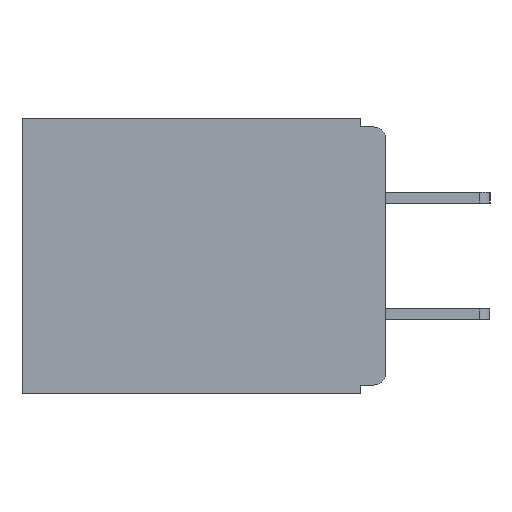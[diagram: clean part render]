
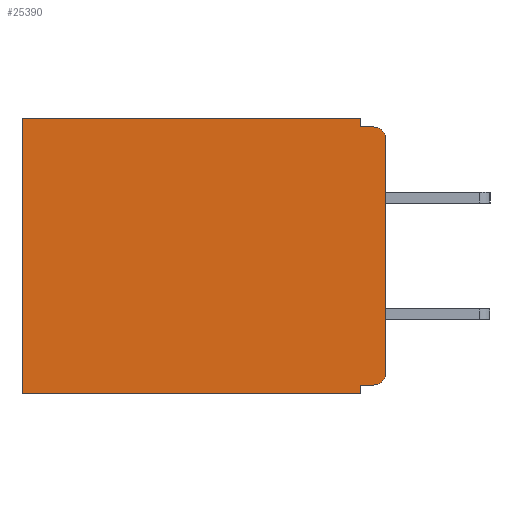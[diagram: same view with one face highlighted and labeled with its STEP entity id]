
A CAD part, left-side view. The second image highlights one B-rep face of the part: STEP entity #25390.
In plain terms, the highlighted planar face has unit normal (-1, 0, 0).
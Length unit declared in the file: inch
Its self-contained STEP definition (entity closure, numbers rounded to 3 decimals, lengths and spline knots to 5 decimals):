
#150 = DIRECTION ( 'NONE',  ( 0., 0., -1. ) ) ;
#1363 = VERTEX_POINT ( 'NONE', #24189 ) ;
#1389 = EDGE_CURVE ( 'NONE', #25102, #22044, #20073, .T. ) ;
#1518 = ORIENTED_EDGE ( 'NONE', *, *, #18378, .T. ) ;
#1550 = EDGE_CURVE ( 'NONE', #19092, #3243, #11316, .T. ) ;
#2679 = DIRECTION ( 'NONE',  ( 1., 0., 0. ) ) ;
#3073 = LINE ( 'NONE', #3217, #8347 ) ;
#3217 = CARTESIAN_POINT ( 'NONE',  ( 0.3, 0., -0.32 ) ) ;
#3243 = VERTEX_POINT ( 'NONE', #17066 ) ;
#3427 = VERTEX_POINT ( 'NONE', #26050 ) ;
#3461 = CIRCLE ( 'NONE', #15539, 0.015 ) ;
#4705 = CARTESIAN_POINT ( 'NONE',  ( 0.3, 0.015, -0.305 ) ) ;
#5525 = DIRECTION ( 'NONE',  ( 0., 1., 0. ) ) ;
#5981 = ORIENTED_EDGE ( 'NONE', *, *, #15393, .T. ) ;
#6112 = VECTOR ( 'NONE', #9221, 39.37008 ) ;
#6397 = DIRECTION ( 'NONE',  ( -1., 0., 0. ) ) ;
#6559 = ORIENTED_EDGE ( 'NONE', *, *, #17235, .T. ) ;
#6800 = CARTESIAN_POINT ( 'NONE',  ( 0.3, 0.031, -0.33 ) ) ;
#6948 = DIRECTION ( 'NONE',  ( 0., 0., -1. ) ) ;
#6993 = CARTESIAN_POINT ( 'NONE',  ( 0.3, 0.031, -0.33 ) ) ;
#8211 = VECTOR ( 'NONE', #22228, 39.37008 ) ;
#8312 = ORIENTED_EDGE ( 'NONE', *, *, #10514, .T. ) ;
#8347 = VECTOR ( 'NONE', #5525, 39.37008 ) ;
#8476 = LINE ( 'NONE', #28039, #12983 ) ;
#9221 = DIRECTION ( 'NONE',  ( 0., 0., -1. ) ) ;
#9336 = PLANE ( 'NONE',  #20077 ) ;
#9478 = AXIS2_PLACEMENT_3D ( 'NONE', #19740, #6397, #22077 ) ;
#9579 = ORIENTED_EDGE ( 'NONE', *, *, #1550, .F. ) ;
#10384 = EDGE_CURVE ( 'NONE', #3427, #17734, #20816, .T. ) ;
#10514 = EDGE_CURVE ( 'NONE', #22943, #13027, #22592, .T. ) ;
#10886 = ORIENTED_EDGE ( 'NONE', *, *, #22960, .F. ) ;
#11005 = CIRCLE ( 'NONE', #9478, 0.015 ) ;
#11316 = LINE ( 'NONE', #28404, #27079 ) ;
#11422 = CARTESIAN_POINT ( 'NONE',  ( 0.3, 0.031, -0.32 ) ) ;
#11884 = CARTESIAN_POINT ( 'NONE',  ( 0.3, 0., 0. ) ) ;
#12770 = ORIENTED_EDGE ( 'NONE', *, *, #20087, .F. ) ;
#12983 = VECTOR ( 'NONE', #16851, 39.37008 ) ;
#13027 = VERTEX_POINT ( 'NONE', #20450 ) ;
#14117 = DIRECTION ( 'NONE',  ( 0., 1., 0. ) ) ;
#14139 = FACE_OUTER_BOUND ( 'NONE', #27091, .T. ) ;
#14296 = DIRECTION ( 'NONE',  ( 0., 1., 0. ) ) ;
#15393 = EDGE_CURVE ( 'NONE', #1363, #17734, #3461, .T. ) ;
#15539 = AXIS2_PLACEMENT_3D ( 'NONE', #4705, #20328, #6948 ) ;
#15869 = DIRECTION ( 'NONE',  ( 0., 0., -1. ) ) ;
#16043 = CARTESIAN_POINT ( 'NONE',  ( 0.3, 0., -0.33 ) ) ;
#16165 = CARTESIAN_POINT ( 'NONE',  ( 0.3, 0., -0.01 ) ) ;
#16545 = VECTOR ( 'NONE', #14117, 39.37008 ) ;
#16851 = DIRECTION ( 'NONE',  ( 0., 0., -1. ) ) ;
#17066 = CARTESIAN_POINT ( 'NONE',  ( 0.3, 0.437, -0.33 ) ) ;
#17235 = EDGE_CURVE ( 'NONE', #13027, #3243, #24314, .T. ) ;
#17734 = VERTEX_POINT ( 'NONE', #26464 ) ;
#18271 = DIRECTION ( 'NONE',  ( 0., 0., -1. ) ) ;
#18378 = EDGE_CURVE ( 'NONE', #3427, #22044, #11005, .T. ) ;
#18539 = EDGE_CURVE ( 'NONE', #19829, #19092, #23931, .T. ) ;
#19092 = VERTEX_POINT ( 'NONE', #6800 ) ;
#19740 = CARTESIAN_POINT ( 'NONE',  ( 0.3, 0.015, -0.025 ) ) ;
#19829 = VERTEX_POINT ( 'NONE', #11422 ) ;
#19998 = ORIENTED_EDGE ( 'NONE', *, *, #18539, .F. ) ;
#20073 = LINE ( 'NONE', #16165, #8211 ) ;
#20077 = AXIS2_PLACEMENT_3D ( 'NONE', #16043, #2679, #18271 ) ;
#20087 = EDGE_CURVE ( 'NONE', #22943, #25102, #8476, .T. ) ;
#20099 = VECTOR ( 'NONE', #15869, 39.37008 ) ;
#20140 = CARTESIAN_POINT ( 'NONE',  ( 0.3, 0.437, -0.33 ) ) ;
#20328 = DIRECTION ( 'NONE',  ( -1., 0., 0. ) ) ;
#20423 = CARTESIAN_POINT ( 'NONE',  ( 0.3, 0., -0.33 ) ) ;
#20450 = CARTESIAN_POINT ( 'NONE',  ( 0.3, 0.437, 0. ) ) ;
#20816 = LINE ( 'NONE', #20423, #20099 ) ;
#21204 = ORIENTED_EDGE ( 'NONE', *, *, #10384, .F. ) ;
#22044 = VERTEX_POINT ( 'NONE', #24681 ) ;
#22077 = DIRECTION ( 'NONE',  ( 0., 0., -1. ) ) ;
#22228 = DIRECTION ( 'NONE',  ( 0., -1., 0. ) ) ;
#22592 = LINE ( 'NONE', #11884, #16545 ) ;
#22943 = VERTEX_POINT ( 'NONE', #27780 ) ;
#22960 = EDGE_CURVE ( 'NONE', #1363, #19829, #3073, .T. ) ;
#22966 = VECTOR ( 'NONE', #150, 39.37008 ) ;
#23931 = LINE ( 'NONE', #6993, #6112 ) ;
#24189 = CARTESIAN_POINT ( 'NONE',  ( 0.3, 0.015, -0.32 ) ) ;
#24314 = LINE ( 'NONE', #20140, #22966 ) ;
#24681 = CARTESIAN_POINT ( 'NONE',  ( 0.3, 0.015, -0.01 ) ) ;
#25102 = VERTEX_POINT ( 'NONE', #26162 ) ;
#25390 = ADVANCED_FACE ( 'NONE', ( #14139 ), #9336, .F. ) ;
#26050 = CARTESIAN_POINT ( 'NONE',  ( 0.3, 0., -0.025 ) ) ;
#26162 = CARTESIAN_POINT ( 'NONE',  ( 0.3, 0.031, -0.01 ) ) ;
#26464 = CARTESIAN_POINT ( 'NONE',  ( 0.3, 0., -0.305 ) ) ;
#27079 = VECTOR ( 'NONE', #14296, 39.37008 ) ;
#27091 = EDGE_LOOP ( 'NONE', ( #21204, #1518, #28333, #12770, #8312, #6559, #9579, #19998, #10886, #5981 ) ) ;
#27780 = CARTESIAN_POINT ( 'NONE',  ( 0.3, 0.031, 0. ) ) ;
#28039 = CARTESIAN_POINT ( 'NONE',  ( 0.3, 0.031, 0. ) ) ;
#28333 = ORIENTED_EDGE ( 'NONE', *, *, #1389, .F. ) ;
#28404 = CARTESIAN_POINT ( 'NONE',  ( 0.3, 0., -0.33 ) ) ;
